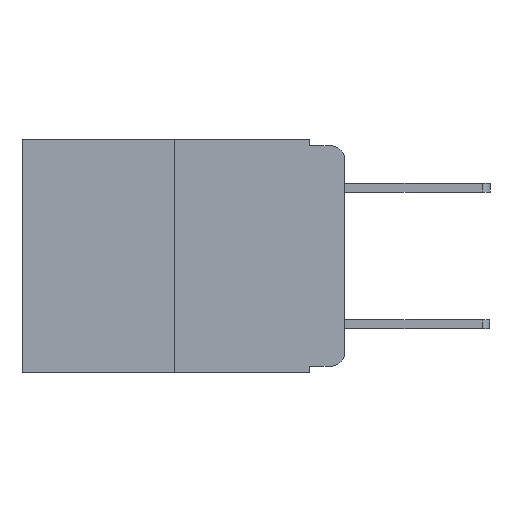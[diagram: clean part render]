
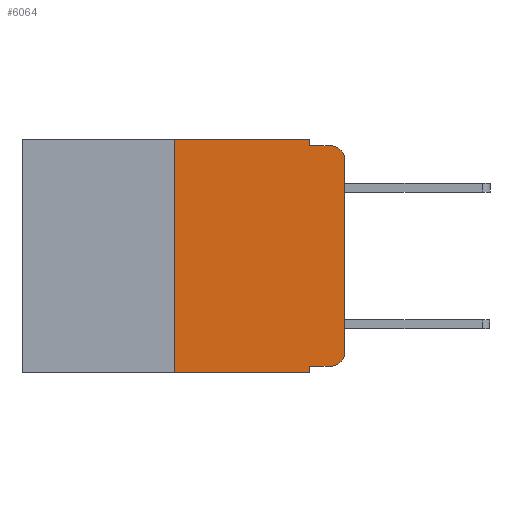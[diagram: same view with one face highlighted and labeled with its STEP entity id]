
A CAD part, left-side view. The second image highlights one B-rep face of the part: STEP entity #6064.
In plain terms, the highlighted planar face has unit normal (-1, 0, 0).
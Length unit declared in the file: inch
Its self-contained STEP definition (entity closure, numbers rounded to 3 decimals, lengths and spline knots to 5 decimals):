
#3 = ORIENTED_EDGE ( 'NONE', *, *, #11481, .F. ) ;
#56 = VERTEX_POINT ( 'NONE', #5674 ) ;
#109 = VERTEX_POINT ( 'NONE', #1263 ) ;
#197 = ORIENTED_EDGE ( 'NONE', *, *, #5987, .F. ) ;
#381 = ORIENTED_EDGE ( 'NONE', *, *, #11930, .T. ) ;
#554 = EDGE_CURVE ( 'NONE', #10929, #2787, #3223, .T. ) ;
#574 = ORIENTED_EDGE ( 'NONE', *, *, #7002, .T. ) ;
#869 = VECTOR ( 'NONE', #1104, 39.37008 ) ;
#1104 = DIRECTION ( 'NONE',  ( 0., 0., -1. ) ) ;
#1160 = LINE ( 'NONE', #1667, #8464 ) ;
#1162 = ORIENTED_EDGE ( 'NONE', *, *, #8861, .T. ) ;
#1205 = LINE ( 'NONE', #1695, #10540 ) ;
#1263 = CARTESIAN_POINT ( 'NONE',  ( 0., 0.02, -0.01 ) ) ;
#1429 = EDGE_CURVE ( 'NONE', #9247, #56, #1160, .T. ) ;
#1667 = CARTESIAN_POINT ( 'NONE',  ( 0., 0.051, -0.333 ) ) ;
#1695 = CARTESIAN_POINT ( 'NONE',  ( 0., 0.051, -0.01 ) ) ;
#1757 = CARTESIAN_POINT ( 'NONE',  ( 0., 0.051, -0.343 ) ) ;
#1917 = ORIENTED_EDGE ( 'NONE', *, *, #2846, .F. ) ;
#1957 = LINE ( 'NONE', #3363, #4559 ) ;
#2260 = ORIENTED_EDGE ( 'NONE', *, *, #554, .F. ) ;
#2300 = CARTESIAN_POINT ( 'NONE',  ( 0., 0.051, 0. ) ) ;
#2408 = VECTOR ( 'NONE', #6476, 39.37008 ) ;
#2595 = VERTEX_POINT ( 'NONE', #8704 ) ;
#2653 = DIRECTION ( 'NONE',  ( 0., -1., 0. ) ) ;
#2661 = AXIS2_PLACEMENT_3D ( 'NONE', #5511, #11743, #3616 ) ;
#2787 = VERTEX_POINT ( 'NONE', #11913 ) ;
#2819 = CARTESIAN_POINT ( 'NONE',  ( 0., 0.473, 0. ) ) ;
#2846 = EDGE_CURVE ( 'NONE', #2595, #10929, #4458, .T. ) ;
#2918 = LINE ( 'NONE', #4971, #9983 ) ;
#3003 = CARTESIAN_POINT ( 'NONE',  ( 0., 0.473, 0. ) ) ;
#3223 = LINE ( 'NONE', #2300, #869 ) ;
#3272 = EDGE_CURVE ( 'NONE', #56, #6810, #9064, .T. ) ;
#3313 = DIRECTION ( 'NONE',  ( -1., 0., 0. ) ) ;
#3363 = CARTESIAN_POINT ( 'NONE',  ( 0., 0.473, -0.343 ) ) ;
#3616 = DIRECTION ( 'NONE',  ( 0., 0., -1. ) ) ;
#3817 = DIRECTION ( 'NONE',  ( 1., 0., 0. ) ) ;
#4030 = DIRECTION ( 'NONE',  ( 0., 0., 1. ) ) ;
#4231 = EDGE_LOOP ( 'NONE', ( #1162, #381, #197, #2260, #1917, #6845, #574, #3, #6987, #5694 ) ) ;
#4458 = LINE ( 'NONE', #3003, #11100 ) ;
#4496 = VERTEX_POINT ( 'NONE', #8224 ) ;
#4559 = VECTOR ( 'NONE', #8084, 39.37008 ) ;
#4963 = CIRCLE ( 'NONE', #11025, 0.02 ) ;
#4971 = CARTESIAN_POINT ( 'NONE',  ( 0., 0.25, 0. ) ) ;
#5511 = CARTESIAN_POINT ( 'NONE',  ( 0., 0.02, -0.313 ) ) ;
#5513 = CARTESIAN_POINT ( 'NONE',  ( 0., 0.051, 0. ) ) ;
#5646 = CARTESIAN_POINT ( 'NONE',  ( 0., 0.051, 0. ) ) ;
#5674 = CARTESIAN_POINT ( 'NONE',  ( 0., 0.02, -0.333 ) ) ;
#5694 = ORIENTED_EDGE ( 'NONE', *, *, #3272, .T. ) ;
#5771 = VERTEX_POINT ( 'NONE', #1757 ) ;
#5987 = EDGE_CURVE ( 'NONE', #2787, #109, #1205, .T. ) ;
#6064 = ADVANCED_FACE ( 'NONE', ( #7673 ), #8443, .F. ) ;
#6476 = DIRECTION ( 'NONE',  ( 0., 0., -1. ) ) ;
#6513 = VECTOR ( 'NONE', #9093, 39.37008 ) ;
#6810 = VERTEX_POINT ( 'NONE', #8727 ) ;
#6845 = ORIENTED_EDGE ( 'NONE', *, *, #9901, .F. ) ;
#6987 = ORIENTED_EDGE ( 'NONE', *, *, #1429, .T. ) ;
#7002 = EDGE_CURVE ( 'NONE', #11117, #5771, #1957, .T. ) ;
#7488 = LINE ( 'NONE', #5513, #2408 ) ;
#7673 = FACE_OUTER_BOUND ( 'NONE', #4231, .T. ) ;
#7825 = CARTESIAN_POINT ( 'NONE',  ( 0., 0.25, -0.343 ) ) ;
#8084 = DIRECTION ( 'NONE',  ( 0., -1., 0. ) ) ;
#8209 = CARTESIAN_POINT ( 'NONE',  ( 0., 0., 0. ) ) ;
#8224 = CARTESIAN_POINT ( 'NONE',  ( 0., 0., -0.03 ) ) ;
#8443 = PLANE ( 'NONE',  #9886 ) ;
#8464 = VECTOR ( 'NONE', #9684, 39.37008 ) ;
#8704 = CARTESIAN_POINT ( 'NONE',  ( 0., 0.25, 0. ) ) ;
#8727 = CARTESIAN_POINT ( 'NONE',  ( 0., 0., -0.313 ) ) ;
#8861 = EDGE_CURVE ( 'NONE', #6810, #4496, #11203, .T. ) ;
#8883 = CARTESIAN_POINT ( 'NONE',  ( 0., 0.02, -0.03 ) ) ;
#9064 = CIRCLE ( 'NONE', #2661, 0.02 ) ;
#9093 = DIRECTION ( 'NONE',  ( 0., 0., 1. ) ) ;
#9247 = VERTEX_POINT ( 'NONE', #10412 ) ;
#9444 = DIRECTION ( 'NONE',  ( 0., -1., 0. ) ) ;
#9684 = DIRECTION ( 'NONE',  ( 0., -1., 0. ) ) ;
#9748 = DIRECTION ( 'NONE',  ( 0., 0., -1. ) ) ;
#9886 = AXIS2_PLACEMENT_3D ( 'NONE', #2819, #3817, #10197 ) ;
#9901 = EDGE_CURVE ( 'NONE', #11117, #2595, #2918, .T. ) ;
#9983 = VECTOR ( 'NONE', #4030, 39.37008 ) ;
#10197 = DIRECTION ( 'NONE',  ( 0., 0., -1. ) ) ;
#10412 = CARTESIAN_POINT ( 'NONE',  ( 0., 0.051, -0.333 ) ) ;
#10540 = VECTOR ( 'NONE', #2653, 39.37008 ) ;
#10929 = VERTEX_POINT ( 'NONE', #5646 ) ;
#11025 = AXIS2_PLACEMENT_3D ( 'NONE', #8883, #3313, #9748 ) ;
#11100 = VECTOR ( 'NONE', #9444, 39.37008 ) ;
#11117 = VERTEX_POINT ( 'NONE', #7825 ) ;
#11203 = LINE ( 'NONE', #8209, #6513 ) ;
#11481 = EDGE_CURVE ( 'NONE', #9247, #5771, #7488, .T. ) ;
#11743 = DIRECTION ( 'NONE',  ( -1., 0., 0. ) ) ;
#11913 = CARTESIAN_POINT ( 'NONE',  ( 0., 0.051, -0.01 ) ) ;
#11930 = EDGE_CURVE ( 'NONE', #4496, #109, #4963, .T. ) ;
